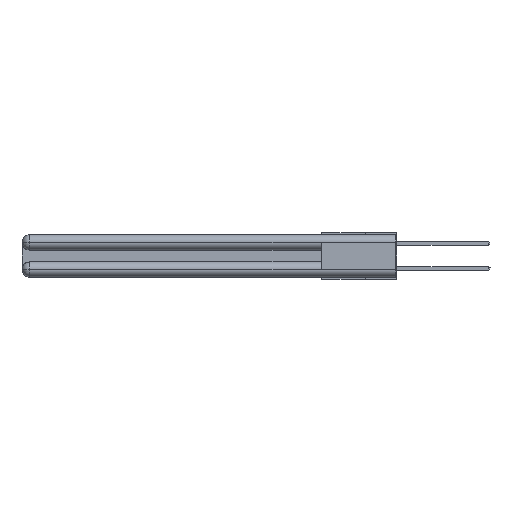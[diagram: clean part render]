
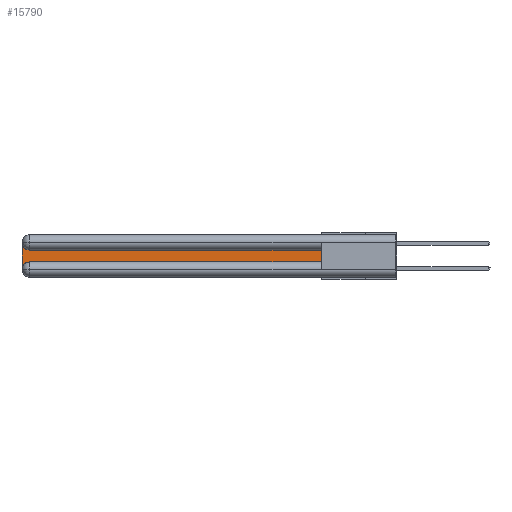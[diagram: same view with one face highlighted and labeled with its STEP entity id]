
A CAD part, left-side view. The second image highlights one B-rep face of the part: STEP entity #15790.
In plain terms, the highlighted planar face has unit normal (-1, 0, 0).
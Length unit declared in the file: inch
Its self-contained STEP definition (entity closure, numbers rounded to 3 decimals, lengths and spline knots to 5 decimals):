
#530 = LINE ( 'NONE', #32178, #32331 ) ;
#673 = VERTEX_POINT ( 'NONE', #16952 ) ;
#1382 = ORIENTED_EDGE ( 'NONE', *, *, #11686, .T. ) ;
#1451 = CARTESIAN_POINT ( 'NONE',  ( 0.075, 0.6, -0.1225 ) ) ;
#3923 = ORIENTED_EDGE ( 'NONE', *, *, #29776, .T. ) ;
#5084 = VERTEX_POINT ( 'NONE', #7724 ) ;
#5348 = CIRCLE ( 'NONE', #24053, 0.06 ) ;
#6041 = DIRECTION ( 'NONE',  ( 0., -1., 0. ) ) ;
#6743 = DIRECTION ( 'NONE',  ( 0., 0., -1. ) ) ;
#7188 = ORIENTED_EDGE ( 'NONE', *, *, #9351, .T. ) ;
#7298 = AXIS2_PLACEMENT_3D ( 'NONE', #22902, #7334, #30894 ) ;
#7334 = DIRECTION ( 'NONE',  ( 1., 0., 0. ) ) ;
#7724 = CARTESIAN_POINT ( 'NONE',  ( 0.075, 0.6, -0.2175 ) ) ;
#8034 = EDGE_CURVE ( 'NONE', #5084, #673, #530, .T. ) ;
#9351 = EDGE_CURVE ( 'NONE', #25592, #11472, #5348, .T. ) ;
#9960 = DIRECTION ( 'NONE',  ( 1., 0., 0. ) ) ;
#10445 = LINE ( 'NONE', #10929, #27102 ) ;
#10929 = CARTESIAN_POINT ( 'NONE',  ( 0.075, 3., -0.2175 ) ) ;
#11472 = VERTEX_POINT ( 'NONE', #30011 ) ;
#11686 = EDGE_CURVE ( 'NONE', #22789, #24268, #13480, .T. ) ;
#12487 = ORIENTED_EDGE ( 'NONE', *, *, #25629, .T. ) ;
#13480 = CIRCLE ( 'NONE', #7298, 0.06 ) ;
#14412 = LINE ( 'NONE', #26761, #17254 ) ;
#14929 = PLANE ( 'NONE',  #19619 ) ;
#15790 = ADVANCED_FACE ( 'NONE', ( #20484 ), #14929, .F. ) ;
#16952 = CARTESIAN_POINT ( 'NONE',  ( 0.075, 0.6, -0.1225 ) ) ;
#16968 = CARTESIAN_POINT ( 'NONE',  ( 0.075, 2.94, -0.0625 ) ) ;
#17019 = ORIENTED_EDGE ( 'NONE', *, *, #33239, .T. ) ;
#17254 = VECTOR ( 'NONE', #6041, 39.37008 ) ;
#17885 = CARTESIAN_POINT ( 'NONE',  ( 0.075, 3., -0.1225 ) ) ;
#19619 = AXIS2_PLACEMENT_3D ( 'NONE', #17885, #9960, #27826 ) ;
#19833 = LINE ( 'NONE', #1451, #27192 ) ;
#20484 = FACE_OUTER_BOUND ( 'NONE', #22170, .T. ) ;
#21567 = DIRECTION ( 'NONE',  ( 0., 0., -1. ) ) ;
#22073 = DIRECTION ( 'NONE',  ( 1., 0., 0. ) ) ;
#22170 = EDGE_LOOP ( 'NONE', ( #17019, #7188, #12487, #1382, #3923, #26274 ) ) ;
#22789 = VERTEX_POINT ( 'NONE', #24644 ) ;
#22902 = CARTESIAN_POINT ( 'NONE',  ( 0.075, 2.94, -0.2775 ) ) ;
#23923 = CARTESIAN_POINT ( 'NONE',  ( 0.075, 2.94, -0.2175 ) ) ;
#24053 = AXIS2_PLACEMENT_3D ( 'NONE', #16968, #22073, #6743 ) ;
#24268 = VERTEX_POINT ( 'NONE', #23923 ) ;
#24644 = CARTESIAN_POINT ( 'NONE',  ( 0.075, 3., -0.2775 ) ) ;
#25592 = VERTEX_POINT ( 'NONE', #29566 ) ;
#25629 = EDGE_CURVE ( 'NONE', #11472, #22789, #10445, .T. ) ;
#26274 = ORIENTED_EDGE ( 'NONE', *, *, #8034, .T. ) ;
#26761 = CARTESIAN_POINT ( 'NONE',  ( 0.075, 0.6, -0.2175 ) ) ;
#27102 = VECTOR ( 'NONE', #21567, 39.37008 ) ;
#27192 = VECTOR ( 'NONE', #30153, 39.37008 ) ;
#27826 = DIRECTION ( 'NONE',  ( 0., 0., -1. ) ) ;
#29454 = DIRECTION ( 'NONE',  ( 0., 0., 1. ) ) ;
#29566 = CARTESIAN_POINT ( 'NONE',  ( 0.075, 2.94, -0.1225 ) ) ;
#29776 = EDGE_CURVE ( 'NONE', #24268, #5084, #14412, .T. ) ;
#30011 = CARTESIAN_POINT ( 'NONE',  ( 0.075, 3., -0.0625 ) ) ;
#30153 = DIRECTION ( 'NONE',  ( 0., 1., 0. ) ) ;
#30894 = DIRECTION ( 'NONE',  ( 0., 0., -1. ) ) ;
#32178 = CARTESIAN_POINT ( 'NONE',  ( 0.075, 0.6, -0.2175 ) ) ;
#32331 = VECTOR ( 'NONE', #29454, 39.37008 ) ;
#33239 = EDGE_CURVE ( 'NONE', #673, #25592, #19833, .T. ) ;
